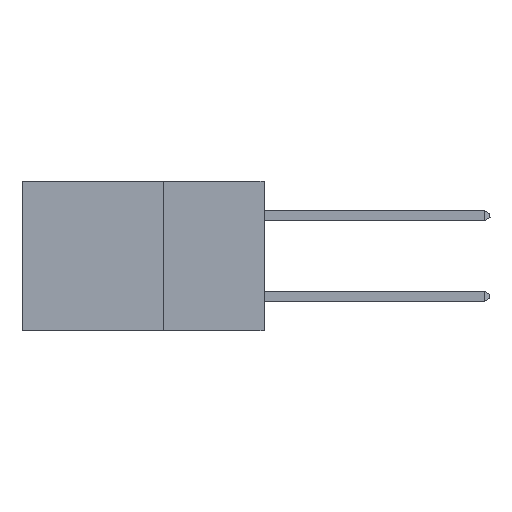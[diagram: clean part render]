
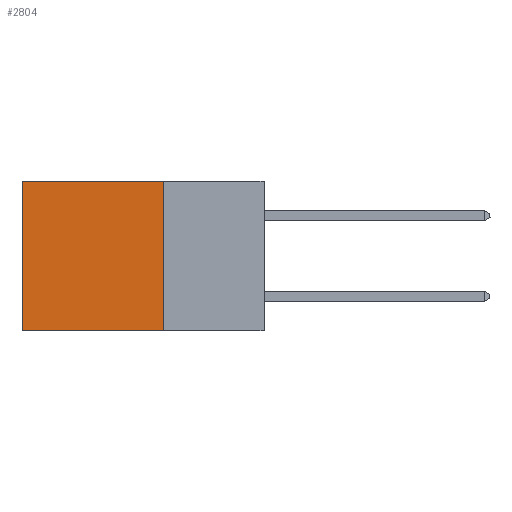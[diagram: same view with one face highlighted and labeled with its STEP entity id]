
A CAD part, left-side view. The second image highlights one B-rep face of the part: STEP entity #2804.
In plain terms, the highlighted planar face has unit normal (-1, 0, 0).
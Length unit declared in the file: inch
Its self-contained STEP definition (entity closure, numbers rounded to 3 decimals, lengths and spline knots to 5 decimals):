
#205 = VERTEX_POINT ( 'NONE', #7234 ) ;
#228 = AXIS2_PLACEMENT_3D ( 'NONE', #5479, #4328, #1831 ) ;
#1075 = DIRECTION ( 'NONE',  ( 0., 0., -1. ) ) ;
#1686 = PLANE ( 'NONE',  #228 ) ;
#1831 = DIRECTION ( 'NONE',  ( 0., 0., -1. ) ) ;
#2654 = ORIENTED_EDGE ( 'NONE', *, *, #11558, .T. ) ;
#2804 = ADVANCED_FACE ( 'NONE', ( #13344 ), #1686, .F. ) ;
#3218 = CARTESIAN_POINT ( 'NONE',  ( 0.298, 0.25, 0. ) ) ;
#3340 = VECTOR ( 'NONE', #3364, 39.37008 ) ;
#3364 = DIRECTION ( 'NONE',  ( 0., 1., 0. ) ) ;
#4328 = DIRECTION ( 'NONE',  ( 1., 0., 0. ) ) ;
#4979 = ORIENTED_EDGE ( 'NONE', *, *, #12015, .F. ) ;
#5058 = EDGE_CURVE ( 'NONE', #205, #6878, #8687, .T. ) ;
#5479 = CARTESIAN_POINT ( 'NONE',  ( 0.298, 0.25, 0. ) ) ;
#5891 = ORIENTED_EDGE ( 'NONE', *, *, #5058, .F. ) ;
#6878 = VERTEX_POINT ( 'NONE', #10041 ) ;
#7234 = CARTESIAN_POINT ( 'NONE',  ( 0.298, 0.25, -0.37 ) ) ;
#7609 = EDGE_CURVE ( 'NONE', #8812, #10085, #11053, .T. ) ;
#8384 = CARTESIAN_POINT ( 'NONE',  ( 0.298, 0.25, 0. ) ) ;
#8687 = LINE ( 'NONE', #9356, #3340 ) ;
#8793 = CARTESIAN_POINT ( 'NONE',  ( 0.298, 0.25, 0. ) ) ;
#8812 = VERTEX_POINT ( 'NONE', #3218 ) ;
#9356 = CARTESIAN_POINT ( 'NONE',  ( 0.298, 0.25, -0.37 ) ) ;
#9534 = VECTOR ( 'NONE', #1075, 39.37008 ) ;
#9618 = CARTESIAN_POINT ( 'NONE',  ( 0.298, 0.6, 0. ) ) ;
#10041 = CARTESIAN_POINT ( 'NONE',  ( 0.298, 0.6, -0.37 ) ) ;
#10078 = LINE ( 'NONE', #8384, #15023 ) ;
#10085 = VERTEX_POINT ( 'NONE', #13592 ) ;
#10860 = VECTOR ( 'NONE', #12219, 39.37008 ) ;
#11053 = LINE ( 'NONE', #8793, #10860 ) ;
#11185 = DIRECTION ( 'NONE',  ( 0., 0., -1. ) ) ;
#11558 = EDGE_CURVE ( 'NONE', #10085, #6878, #15408, .T. ) ;
#12015 = EDGE_CURVE ( 'NONE', #8812, #205, #10078, .T. ) ;
#12219 = DIRECTION ( 'NONE',  ( 0., 1., 0. ) ) ;
#13344 = FACE_OUTER_BOUND ( 'NONE', #13883, .T. ) ;
#13592 = CARTESIAN_POINT ( 'NONE',  ( 0.298, 0.6, 0. ) ) ;
#13883 = EDGE_LOOP ( 'NONE', ( #2654, #5891, #4979, #14583 ) ) ;
#14583 = ORIENTED_EDGE ( 'NONE', *, *, #7609, .T. ) ;
#15023 = VECTOR ( 'NONE', #11185, 39.37008 ) ;
#15408 = LINE ( 'NONE', #9618, #9534 ) ;
